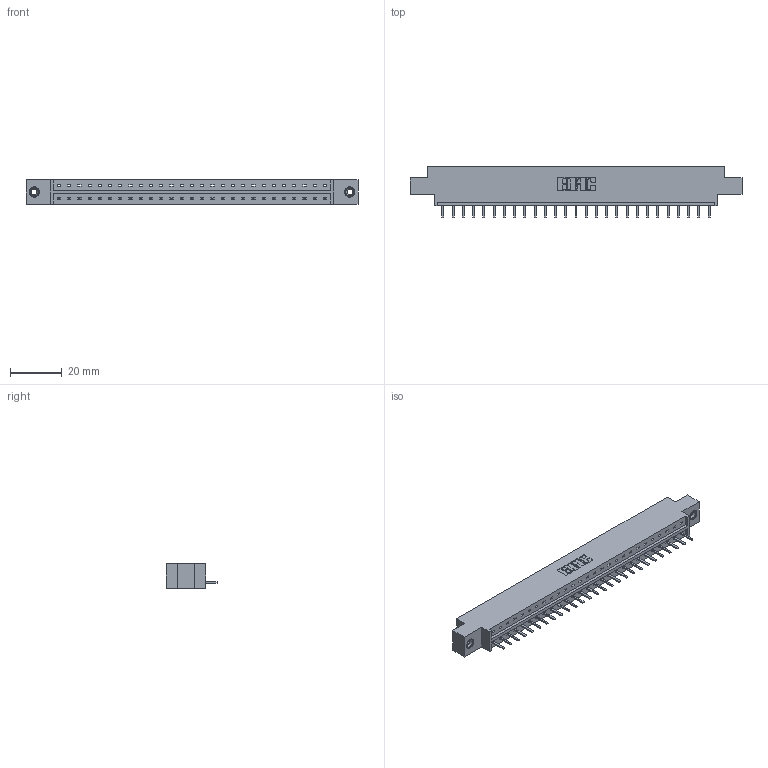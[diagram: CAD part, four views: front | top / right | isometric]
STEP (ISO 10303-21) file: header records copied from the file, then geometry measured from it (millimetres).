
FILE_DESCRIPTION (( 'STEP AP203' ), '1' );
FILE_NAME ('333-027-520-608.STEP', '2018-08-02T13:46:40', ( '' ), ( '' ), 'SwSTEP 2.0', 'SolidWorks 2016', '' );
FILE_SCHEMA (( 'CONFIG_CONTROL_DESIGN' ));
Length unit declared in the file: inch
Products named in the file (4): 333 Part_Offset - .156 Dia - TI; 345-292-001_345-293-120; 345-250-001_345-250-003-102; 333-027-520-608
Assembly tree (30 placements, depth 2):
  333-027-520-608
    333 Part_Offset - .156 Dia - TI
    345-292-001_345-293-120  x27
    345-250-001_345-250-003-102  x2
Bounding box: 128.52 x 20.02 x 9.4 mm (x, y, z)
Volume: 12492.2 mm3; surface area: 13369.5 mm2
Topology: 30 solids, 30 shells, 1852 faces, 5427 edges, 3538 vertices
Faces by surface type: plane 1294, cylinder 542, cone 12, torus 4
Entity records: 19878 total; most frequent: CARTESIAN_POINT 3426, ORIENTED_EDGE 3370, DIRECTION 2941, EDGE_CURVE 1685, VECTOR 1533, LINE 1533, VERTEX_POINT 1116, AXIS2_PLACEMENT_3D 704
